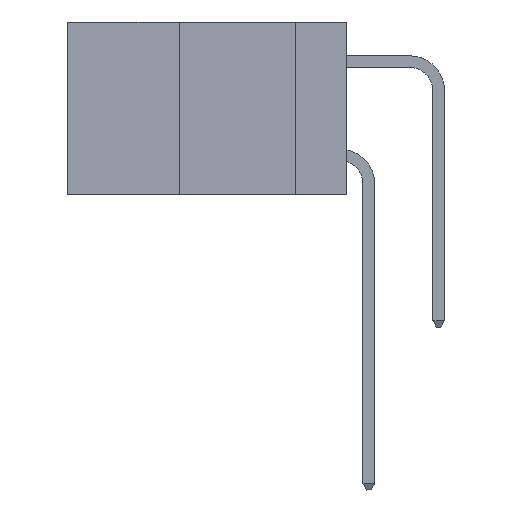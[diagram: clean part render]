
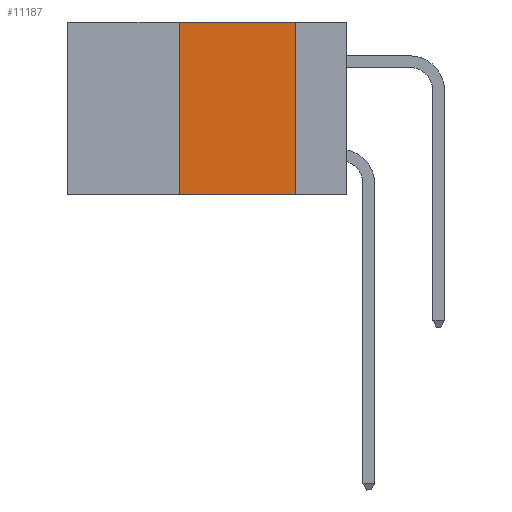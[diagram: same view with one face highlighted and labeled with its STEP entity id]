
A CAD part, left-side view. The second image highlights one B-rep face of the part: STEP entity #11187.
In plain terms, the highlighted planar face has unit normal (-1, 0, 0).
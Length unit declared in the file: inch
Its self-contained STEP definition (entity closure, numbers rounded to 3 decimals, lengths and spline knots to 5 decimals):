
#2384 = LINE ( 'NONE', #35008, #4171 ) ;
#2567 = ORIENTED_EDGE ( 'NONE', *, *, #31695, .F. ) ;
#2976 = CARTESIAN_POINT ( 'NONE',  ( 0., 0.36, -0.37 ) ) ;
#4171 = VECTOR ( 'NONE', #14457, 39.37008 ) ;
#4352 = DIRECTION ( 'NONE',  ( 0., 0., -1. ) ) ;
#8238 = EDGE_CURVE ( 'NONE', #36866, #33553, #22130, .T. ) ;
#10421 = VECTOR ( 'NONE', #34189, 39.37008 ) ;
#10870 = VERTEX_POINT ( 'NONE', #30915 ) ;
#11187 = ADVANCED_FACE ( 'NONE', ( #16618 ), #19982, .F. ) ;
#12994 = CARTESIAN_POINT ( 'NONE',  ( 0., 0.11, -0.37 ) ) ;
#14457 = DIRECTION ( 'NONE',  ( 0., 0., 1. ) ) ;
#15554 = LINE ( 'NONE', #26835, #31032 ) ;
#16218 = VERTEX_POINT ( 'NONE', #2976 ) ;
#16618 = FACE_OUTER_BOUND ( 'NONE', #32616, .T. ) ;
#18516 = DIRECTION ( 'NONE',  ( 0., -1., 0. ) ) ;
#19982 = PLANE ( 'NONE',  #23847 ) ;
#20834 = CARTESIAN_POINT ( 'NONE',  ( 0., 0.6, 0. ) ) ;
#21121 = EDGE_CURVE ( 'NONE', #16218, #33553, #15554, .T. ) ;
#22130 = LINE ( 'NONE', #37916, #10421 ) ;
#22349 = ORIENTED_EDGE ( 'NONE', *, *, #36907, .F. ) ;
#22749 = DIRECTION ( 'NONE',  ( 1., 0., 0. ) ) ;
#22767 = CARTESIAN_POINT ( 'NONE',  ( 0., 0.11, 0. ) ) ;
#23847 = AXIS2_PLACEMENT_3D ( 'NONE', #34987, #22749, #4352 ) ;
#26835 = CARTESIAN_POINT ( 'NONE',  ( 0., 0.6, -0.37 ) ) ;
#29738 = DIRECTION ( 'NONE',  ( 0., -1., 0. ) ) ;
#30915 = CARTESIAN_POINT ( 'NONE',  ( 0., 0.36, 0. ) ) ;
#31032 = VECTOR ( 'NONE', #18516, 39.37008 ) ;
#31144 = VECTOR ( 'NONE', #29738, 39.37008 ) ;
#31695 = EDGE_CURVE ( 'NONE', #10870, #36866, #38433, .T. ) ;
#32616 = EDGE_LOOP ( 'NONE', ( #35967, #2567, #22349, #33428 ) ) ;
#33428 = ORIENTED_EDGE ( 'NONE', *, *, #21121, .T. ) ;
#33553 = VERTEX_POINT ( 'NONE', #12994 ) ;
#34189 = DIRECTION ( 'NONE',  ( 0., 0., -1. ) ) ;
#34987 = CARTESIAN_POINT ( 'NONE',  ( 0., 0.6, 0. ) ) ;
#35008 = CARTESIAN_POINT ( 'NONE',  ( 0., 0.36, 0. ) ) ;
#35967 = ORIENTED_EDGE ( 'NONE', *, *, #8238, .F. ) ;
#36866 = VERTEX_POINT ( 'NONE', #22767 ) ;
#36907 = EDGE_CURVE ( 'NONE', #16218, #10870, #2384, .T. ) ;
#37916 = CARTESIAN_POINT ( 'NONE',  ( 0., 0.11, 0. ) ) ;
#38433 = LINE ( 'NONE', #20834, #31144 ) ;
